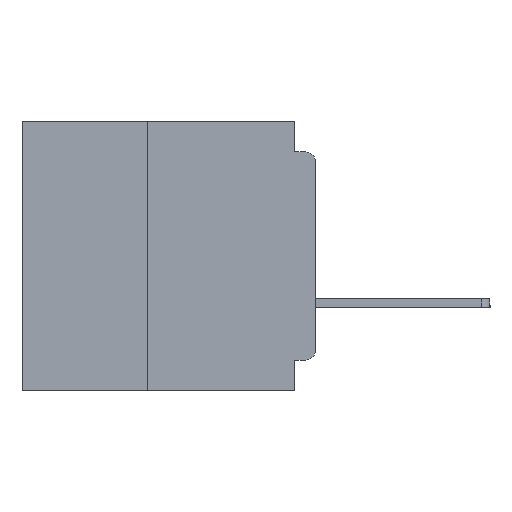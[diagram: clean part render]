
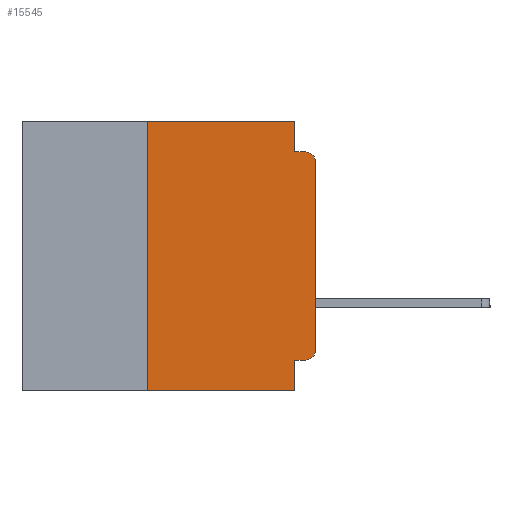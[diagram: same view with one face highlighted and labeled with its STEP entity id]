
A CAD part, left-side view. The second image highlights one B-rep face of the part: STEP entity #15545.
In plain terms, the highlighted planar face has unit normal (-1, 0, 0).
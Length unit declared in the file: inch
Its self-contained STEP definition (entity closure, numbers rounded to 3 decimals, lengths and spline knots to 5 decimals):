
#1808 = CARTESIAN_POINT ( 'NONE',  ( 0., 0.25, -0.4 ) ) ;
#3503 = CARTESIAN_POINT ( 'NONE',  ( 0., 0.437, 0. ) ) ;
#4324 = DIRECTION ( 'NONE',  ( -1., 0., 0. ) ) ;
#5187 = VERTEX_POINT ( 'NONE', #53054 ) ;
#6795 = VECTOR ( 'NONE', #55767, 39.37008 ) ;
#6898 = DIRECTION ( 'NONE',  ( 0., 0., 1. ) ) ;
#6956 = VERTEX_POINT ( 'NONE', #48102 ) ;
#8900 = CARTESIAN_POINT ( 'NONE',  ( 0., 0.031, -0.4 ) ) ;
#9491 = CARTESIAN_POINT ( 'NONE',  ( 0., 0.015, -0.06 ) ) ;
#10214 = CARTESIAN_POINT ( 'NONE',  ( 0., 0.031, -0.045 ) ) ;
#10380 = EDGE_CURVE ( 'NONE', #57265, #32322, #57285, .T. ) ;
#10970 = CARTESIAN_POINT ( 'NONE',  ( 0., 0.031, -0.4 ) ) ;
#12160 = LINE ( 'NONE', #25480, #57157 ) ;
#12389 = ORIENTED_EDGE ( 'NONE', *, *, #26082, .T. ) ;
#12520 = PLANE ( 'NONE',  #32704 ) ;
#13241 = VERTEX_POINT ( 'NONE', #8900 ) ;
#13657 = VECTOR ( 'NONE', #49128, 39.37008 ) ;
#13780 = ORIENTED_EDGE ( 'NONE', *, *, #15338, .F. ) ;
#13850 = CARTESIAN_POINT ( 'NONE',  ( 0., 0., -0.045 ) ) ;
#14000 = DIRECTION ( 'NONE',  ( 0., 0., -1. ) ) ;
#14085 = VECTOR ( 'NONE', #32418, 39.37008 ) ;
#15338 = EDGE_CURVE ( 'NONE', #31759, #13241, #43991, .T. ) ;
#15400 = LINE ( 'NONE', #13850, #49834 ) ;
#15545 = ADVANCED_FACE ( 'NONE', ( #56640 ), #12520, .F. ) ;
#16305 = EDGE_CURVE ( 'NONE', #5187, #31759, #48806, .T. ) ;
#17050 = DIRECTION ( 'NONE',  ( 0., 0., -1. ) ) ;
#17331 = AXIS2_PLACEMENT_3D ( 'NONE', #31235, #4324, #35756 ) ;
#17708 = CARTESIAN_POINT ( 'NONE',  ( 0., 0.437, -0.4 ) ) ;
#18347 = EDGE_CURVE ( 'NONE', #6956, #36455, #26038, .T. ) ;
#19853 = EDGE_CURVE ( 'NONE', #46950, #21831, #15400, .T. ) ;
#21456 = VECTOR ( 'NONE', #6898, 39.37008 ) ;
#21831 = VERTEX_POINT ( 'NONE', #41111 ) ;
#22245 = CARTESIAN_POINT ( 'NONE',  ( 0., 0.031, 0. ) ) ;
#24821 = EDGE_LOOP ( 'NONE', ( #45779, #46304, #51257, #57607, #50310, #31621, #45582, #13780, #54696, #12389 ) ) ;
#25480 = CARTESIAN_POINT ( 'NONE',  ( 0., 0.031, 0. ) ) ;
#25747 = EDGE_CURVE ( 'NONE', #33062, #6956, #35628, .T. ) ;
#25793 = DIRECTION ( 'NONE',  ( 0., 1., 0. ) ) ;
#25927 = CARTESIAN_POINT ( 'NONE',  ( 0., 0.25, -0.4 ) ) ;
#26038 = LINE ( 'NONE', #50313, #14085 ) ;
#26082 = EDGE_CURVE ( 'NONE', #5187, #57265, #42584, .T. ) ;
#26789 = AXIS2_PLACEMENT_3D ( 'NONE', #9491, #40901, #14000 ) ;
#27279 = EDGE_CURVE ( 'NONE', #32322, #21831, #39775, .T. ) ;
#29987 = DIRECTION ( 'NONE',  ( 0., 0., -1. ) ) ;
#31235 = CARTESIAN_POINT ( 'NONE',  ( 0., 0.015, -0.34 ) ) ;
#31621 = ORIENTED_EDGE ( 'NONE', *, *, #25747, .F. ) ;
#31759 = VERTEX_POINT ( 'NONE', #39388 ) ;
#32322 = VERTEX_POINT ( 'NONE', #38936 ) ;
#32418 = DIRECTION ( 'NONE',  ( 0., -1., 0. ) ) ;
#32704 = AXIS2_PLACEMENT_3D ( 'NONE', #3503, #43929, #17050 ) ;
#33062 = VERTEX_POINT ( 'NONE', #25927 ) ;
#35628 = LINE ( 'NONE', #1808, #37006 ) ;
#35756 = DIRECTION ( 'NONE',  ( 0., 0., -1. ) ) ;
#36455 = VERTEX_POINT ( 'NONE', #22245 ) ;
#36855 = VECTOR ( 'NONE', #25793, 39.37008 ) ;
#37006 = VECTOR ( 'NONE', #42053, 39.37008 ) ;
#38936 = CARTESIAN_POINT ( 'NONE',  ( 0., 0., -0.06 ) ) ;
#39388 = CARTESIAN_POINT ( 'NONE',  ( 0., 0.031, -0.355 ) ) ;
#39775 = CIRCLE ( 'NONE', #26789, 0.015 ) ;
#40738 = DIRECTION ( 'NONE',  ( 0., -1., 0. ) ) ;
#40901 = DIRECTION ( 'NONE',  ( -1., 0., 0. ) ) ;
#41111 = CARTESIAN_POINT ( 'NONE',  ( 0., 0.015, -0.045 ) ) ;
#42053 = DIRECTION ( 'NONE',  ( 0., 0., 1. ) ) ;
#42411 = EDGE_CURVE ( 'NONE', #33062, #13241, #50918, .T. ) ;
#42584 = CIRCLE ( 'NONE', #17331, 0.015 ) ;
#43636 = CARTESIAN_POINT ( 'NONE',  ( 0., 0., -0.355 ) ) ;
#43929 = DIRECTION ( 'NONE',  ( 1., 0., 0. ) ) ;
#43991 = LINE ( 'NONE', #10970, #6795 ) ;
#45582 = ORIENTED_EDGE ( 'NONE', *, *, #42411, .T. ) ;
#45779 = ORIENTED_EDGE ( 'NONE', *, *, #10380, .T. ) ;
#46304 = ORIENTED_EDGE ( 'NONE', *, *, #27279, .T. ) ;
#46950 = VERTEX_POINT ( 'NONE', #10214 ) ;
#47370 = EDGE_CURVE ( 'NONE', #36455, #46950, #12160, .T. ) ;
#47792 = CARTESIAN_POINT ( 'NONE',  ( 0., 0., -0.34 ) ) ;
#48102 = CARTESIAN_POINT ( 'NONE',  ( 0., 0.25, 0. ) ) ;
#48806 = LINE ( 'NONE', #43636, #36855 ) ;
#49128 = DIRECTION ( 'NONE',  ( 0., -1., 0. ) ) ;
#49834 = VECTOR ( 'NONE', #40738, 39.37008 ) ;
#50310 = ORIENTED_EDGE ( 'NONE', *, *, #18347, .F. ) ;
#50313 = CARTESIAN_POINT ( 'NONE',  ( 0., 0.437, 0. ) ) ;
#50918 = LINE ( 'NONE', #17708, #13657 ) ;
#51257 = ORIENTED_EDGE ( 'NONE', *, *, #19853, .F. ) ;
#53054 = CARTESIAN_POINT ( 'NONE',  ( 0., 0.015, -0.355 ) ) ;
#54696 = ORIENTED_EDGE ( 'NONE', *, *, #16305, .F. ) ;
#55767 = DIRECTION ( 'NONE',  ( 0., 0., -1. ) ) ;
#56166 = CARTESIAN_POINT ( 'NONE',  ( 0., 0., 0. ) ) ;
#56640 = FACE_OUTER_BOUND ( 'NONE', #24821, .T. ) ;
#57157 = VECTOR ( 'NONE', #29987, 39.37008 ) ;
#57265 = VERTEX_POINT ( 'NONE', #47792 ) ;
#57285 = LINE ( 'NONE', #56166, #21456 ) ;
#57607 = ORIENTED_EDGE ( 'NONE', *, *, #47370, .F. ) ;
